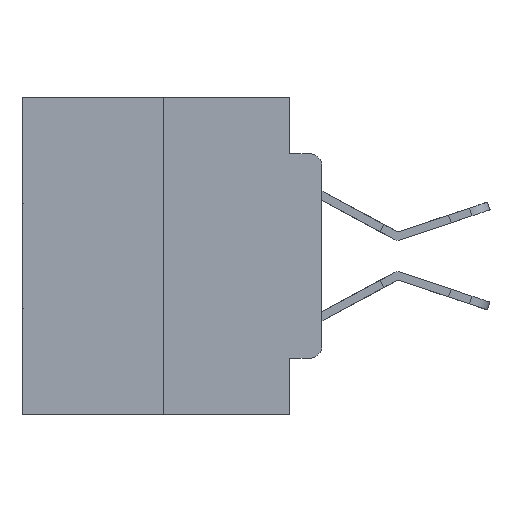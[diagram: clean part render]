
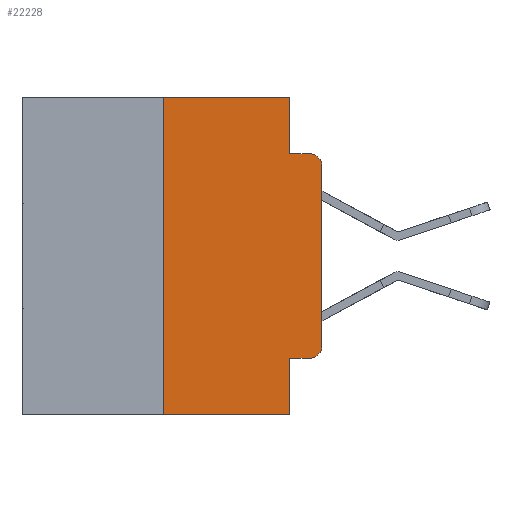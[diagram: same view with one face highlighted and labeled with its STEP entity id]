
A CAD part, left-side view. The second image highlights one B-rep face of the part: STEP entity #22228.
In plain terms, the highlighted planar face has unit normal (-1, 0, 0).
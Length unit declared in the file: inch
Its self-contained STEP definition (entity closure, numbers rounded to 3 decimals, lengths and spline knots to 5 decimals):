
#474 = AXIS2_PLACEMENT_3D ( 'NONE', #19158, #5501, #21430 ) ;
#508 = CARTESIAN_POINT ( 'NONE',  ( 0., 0.473, 0. ) ) ;
#1305 = CARTESIAN_POINT ( 'NONE',  ( 0., 0.25, -0.5 ) ) ;
#1639 = EDGE_LOOP ( 'NONE', ( #10510, #15862, #8730, #9137, #1878, #22624, #22995, #24764, #10139, #24289 ) ) ;
#1878 = ORIENTED_EDGE ( 'NONE', *, *, #21029, .F. ) ;
#2693 = CARTESIAN_POINT ( 'NONE',  ( 0., 0.051, 0. ) ) ;
#3019 = CARTESIAN_POINT ( 'NONE',  ( 0., 0.051, -0.5 ) ) ;
#3364 = VECTOR ( 'NONE', #7171, 39.37008 ) ;
#3392 = LINE ( 'NONE', #7782, #19490 ) ;
#3632 = LINE ( 'NONE', #16410, #27089 ) ;
#5204 = DIRECTION ( 'NONE',  ( 0., 0., -1. ) ) ;
#5497 = VERTEX_POINT ( 'NONE', #5880 ) ;
#5501 = DIRECTION ( 'NONE',  ( -1., 0., 0. ) ) ;
#5858 = EDGE_CURVE ( 'NONE', #5900, #28980, #8830, .T. ) ;
#5880 = CARTESIAN_POINT ( 'NONE',  ( 0., 0.051, -0.0885 ) ) ;
#5900 = VERTEX_POINT ( 'NONE', #9536 ) ;
#6046 = CARTESIAN_POINT ( 'NONE',  ( 0., 0.25, 0. ) ) ;
#6228 = CARTESIAN_POINT ( 'NONE',  ( 0., 0., 0. ) ) ;
#6236 = FACE_OUTER_BOUND ( 'NONE', #1639, .T. ) ;
#7171 = DIRECTION ( 'NONE',  ( 0., -1., 0. ) ) ;
#7294 = DIRECTION ( 'NONE',  ( 0., 0., -1. ) ) ;
#7402 = EDGE_CURVE ( 'NONE', #5900, #11885, #3632, .T. ) ;
#7782 = CARTESIAN_POINT ( 'NONE',  ( 0., 0.473, 0. ) ) ;
#7795 = VECTOR ( 'NONE', #14300, 39.37008 ) ;
#8547 = VERTEX_POINT ( 'NONE', #26922 ) ;
#8567 = DIRECTION ( 'NONE',  ( 0., 0., 1. ) ) ;
#8730 = ORIENTED_EDGE ( 'NONE', *, *, #18115, .F. ) ;
#8830 = LINE ( 'NONE', #20798, #3364 ) ;
#9137 = ORIENTED_EDGE ( 'NONE', *, *, #16613, .F. ) ;
#9221 = AXIS2_PLACEMENT_3D ( 'NONE', #508, #18856, #5204 ) ;
#9536 = CARTESIAN_POINT ( 'NONE',  ( 0., 0.051, -0.4115 ) ) ;
#9728 = DIRECTION ( 'NONE',  ( -1., 0., 0. ) ) ;
#9847 = CARTESIAN_POINT ( 'NONE',  ( 0., 0., -0.1085 ) ) ;
#10139 = ORIENTED_EDGE ( 'NONE', *, *, #5858, .T. ) ;
#10510 = ORIENTED_EDGE ( 'NONE', *, *, #25624, .T. ) ;
#11626 = VERTEX_POINT ( 'NONE', #9847 ) ;
#11854 = VECTOR ( 'NONE', #13561, 39.37008 ) ;
#11885 = VERTEX_POINT ( 'NONE', #3019 ) ;
#12030 = VERTEX_POINT ( 'NONE', #1305 ) ;
#12045 = LINE ( 'NONE', #6046, #29239 ) ;
#12398 = VERTEX_POINT ( 'NONE', #14109 ) ;
#13012 = DIRECTION ( 'NONE',  ( 0., 0., 1. ) ) ;
#13184 = CIRCLE ( 'NONE', #21986, 0.02 ) ;
#13561 = DIRECTION ( 'NONE',  ( 0., -1., 0. ) ) ;
#13921 = LINE ( 'NONE', #27730, #7795 ) ;
#14109 = CARTESIAN_POINT ( 'NONE',  ( 0., 0.02, -0.0885 ) ) ;
#14300 = DIRECTION ( 'NONE',  ( 0., -1., 0. ) ) ;
#14998 = VECTOR ( 'NONE', #8567, 39.37008 ) ;
#15089 = EDGE_CURVE ( 'NONE', #12030, #8547, #12045, .T. ) ;
#15826 = CARTESIAN_POINT ( 'NONE',  ( 0., 0.051, -0.0885 ) ) ;
#15862 = ORIENTED_EDGE ( 'NONE', *, *, #24142, .T. ) ;
#16410 = CARTESIAN_POINT ( 'NONE',  ( 0., 0.051, 0. ) ) ;
#16613 = EDGE_CURVE ( 'NONE', #27287, #5497, #17588, .T. ) ;
#16625 = PLANE ( 'NONE',  #9221 ) ;
#17588 = LINE ( 'NONE', #2693, #26178 ) ;
#18115 = EDGE_CURVE ( 'NONE', #5497, #12398, #23823, .T. ) ;
#18726 = DIRECTION ( 'NONE',  ( 0., 0., -1. ) ) ;
#18856 = DIRECTION ( 'NONE',  ( 1., 0., 0. ) ) ;
#18908 = EDGE_CURVE ( 'NONE', #12030, #11885, #13921, .T. ) ;
#19158 = CARTESIAN_POINT ( 'NONE',  ( 0., 0.02, -0.1085 ) ) ;
#19490 = VECTOR ( 'NONE', #21392, 39.37008 ) ;
#20263 = LINE ( 'NONE', #6228, #14998 ) ;
#20714 = CIRCLE ( 'NONE', #474, 0.02 ) ;
#20798 = CARTESIAN_POINT ( 'NONE',  ( 0., 0.051, -0.4115 ) ) ;
#21029 = EDGE_CURVE ( 'NONE', #8547, #27287, #3392, .T. ) ;
#21392 = DIRECTION ( 'NONE',  ( 0., -1., 0. ) ) ;
#21430 = DIRECTION ( 'NONE',  ( 0., 0., -1. ) ) ;
#21597 = CARTESIAN_POINT ( 'NONE',  ( 0., 0., -0.3915 ) ) ;
#21986 = AXIS2_PLACEMENT_3D ( 'NONE', #23257, #9728, #25499 ) ;
#22228 = ADVANCED_FACE ( 'NONE', ( #6236 ), #16625, .F. ) ;
#22624 = ORIENTED_EDGE ( 'NONE', *, *, #15089, .F. ) ;
#22995 = ORIENTED_EDGE ( 'NONE', *, *, #18908, .T. ) ;
#23076 = CARTESIAN_POINT ( 'NONE',  ( 0., 0.051, 0. ) ) ;
#23257 = CARTESIAN_POINT ( 'NONE',  ( 0., 0.02, -0.3915 ) ) ;
#23823 = LINE ( 'NONE', #15826, #11854 ) ;
#24142 = EDGE_CURVE ( 'NONE', #11626, #12398, #20714, .T. ) ;
#24289 = ORIENTED_EDGE ( 'NONE', *, *, #29169, .T. ) ;
#24764 = ORIENTED_EDGE ( 'NONE', *, *, #7402, .F. ) ;
#24840 = VERTEX_POINT ( 'NONE', #21597 ) ;
#24846 = CARTESIAN_POINT ( 'NONE',  ( 0., 0.02, -0.4115 ) ) ;
#25499 = DIRECTION ( 'NONE',  ( 0., 0., -1. ) ) ;
#25624 = EDGE_CURVE ( 'NONE', #24840, #11626, #20263, .T. ) ;
#26178 = VECTOR ( 'NONE', #18726, 39.37008 ) ;
#26922 = CARTESIAN_POINT ( 'NONE',  ( 0., 0.25, 0. ) ) ;
#27089 = VECTOR ( 'NONE', #7294, 39.37008 ) ;
#27287 = VERTEX_POINT ( 'NONE', #23076 ) ;
#27730 = CARTESIAN_POINT ( 'NONE',  ( 0., 0.473, -0.5 ) ) ;
#28980 = VERTEX_POINT ( 'NONE', #24846 ) ;
#29169 = EDGE_CURVE ( 'NONE', #28980, #24840, #13184, .T. ) ;
#29239 = VECTOR ( 'NONE', #13012, 39.37008 ) ;
